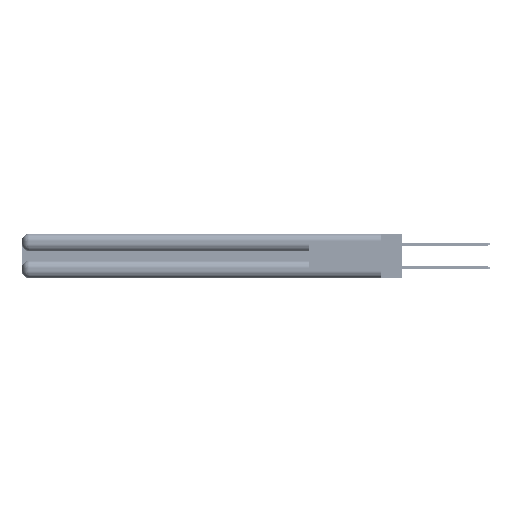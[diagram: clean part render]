
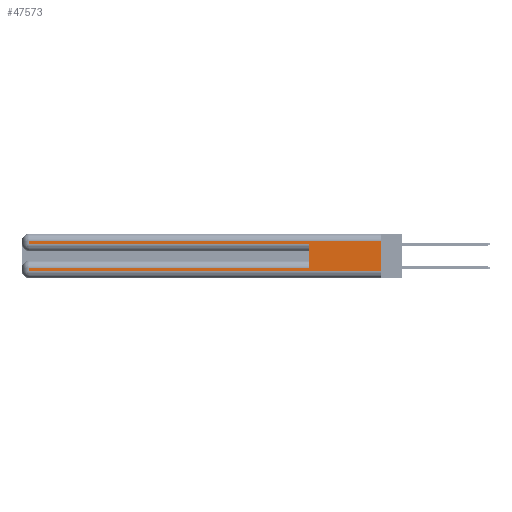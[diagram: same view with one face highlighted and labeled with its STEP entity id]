
A CAD part, left-side view. The second image highlights one B-rep face of the part: STEP entity #47573.
In plain terms, the highlighted planar face has unit normal (-1, 0, 0).
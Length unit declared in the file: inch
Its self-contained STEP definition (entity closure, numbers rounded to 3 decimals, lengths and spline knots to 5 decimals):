
#37 = VECTOR ( 'NONE', #35534, 39.37008 ) ;
#205 = VERTEX_POINT ( 'NONE', #32773 ) ;
#1882 = CARTESIAN_POINT ( 'NONE',  ( 0., 0.6, 0.085 ) ) ;
#2250 = CARTESIAN_POINT ( 'NONE',  ( 0., 2.94, 0.085 ) ) ;
#2563 = EDGE_CURVE ( 'NONE', #205, #37774, #5946, .T. ) ;
#3635 = CARTESIAN_POINT ( 'NONE',  ( 0., 0., 0.285 ) ) ;
#4123 = ORIENTED_EDGE ( 'NONE', *, *, #25211, .F. ) ;
#5076 = VECTOR ( 'NONE', #13682, 39.37008 ) ;
#5824 = EDGE_CURVE ( 'NONE', #36626, #10747, #19608, .T. ) ;
#5946 = LINE ( 'NONE', #14406, #26846 ) ;
#6114 = VERTEX_POINT ( 'NONE', #18124 ) ;
#6304 = CARTESIAN_POINT ( 'NONE',  ( 0., 2.94, 0.37 ) ) ;
#6637 = VECTOR ( 'NONE', #47130, 39.37008 ) ;
#7962 = LINE ( 'NONE', #22402, #6637 ) ;
#8112 = ORIENTED_EDGE ( 'NONE', *, *, #26321, .T. ) ;
#8675 = CARTESIAN_POINT ( 'NONE',  ( 0., 2.94, 0.37 ) ) ;
#10031 = ORIENTED_EDGE ( 'NONE', *, *, #43802, .T. ) ;
#10523 = DIRECTION ( 'NONE',  ( 0., -1., 0. ) ) ;
#10747 = VERTEX_POINT ( 'NONE', #31494 ) ;
#11417 = DIRECTION ( 'NONE',  ( 0., 1., 0. ) ) ;
#12147 = DIRECTION ( 'NONE',  ( 0., -1., 0. ) ) ;
#12159 = LINE ( 'NONE', #44704, #24508 ) ;
#13682 = DIRECTION ( 'NONE',  ( 0., 0., -1. ) ) ;
#13948 = VECTOR ( 'NONE', #46022, 39.37008 ) ;
#14031 = ORIENTED_EDGE ( 'NONE', *, *, #5824, .T. ) ;
#14406 = CARTESIAN_POINT ( 'NONE',  ( 0., 0., 0.06 ) ) ;
#17863 = CARTESIAN_POINT ( 'NONE',  ( 0., 0., 0.37 ) ) ;
#18124 = CARTESIAN_POINT ( 'NONE',  ( 0., 2.94, 0.31 ) ) ;
#19393 = VERTEX_POINT ( 'NONE', #2250 ) ;
#19608 = LINE ( 'NONE', #3635, #30580 ) ;
#19993 = DIRECTION ( 'NONE',  ( 0., 0., 1. ) ) ;
#21186 = ORIENTED_EDGE ( 'NONE', *, *, #26703, .T. ) ;
#22244 = PLANE ( 'NONE',  #25597 ) ;
#22402 = CARTESIAN_POINT ( 'NONE',  ( 0., 0., 0.31 ) ) ;
#22417 = DIRECTION ( 'NONE',  ( 1., 0., 0. ) ) ;
#22661 = CARTESIAN_POINT ( 'NONE',  ( 0., 0., 0.31 ) ) ;
#24508 = VECTOR ( 'NONE', #19993, 39.37008 ) ;
#25211 = EDGE_CURVE ( 'NONE', #25696, #10747, #12159, .T. ) ;
#25597 = AXIS2_PLACEMENT_3D ( 'NONE', #47141, #22417, #51303 ) ;
#25696 = VERTEX_POINT ( 'NONE', #1882 ) ;
#26321 = EDGE_CURVE ( 'NONE', #19393, #205, #33384, .T. ) ;
#26703 = EDGE_CURVE ( 'NONE', #6114, #36626, #46954, .T. ) ;
#26846 = VECTOR ( 'NONE', #10523, 39.37008 ) ;
#28948 = ORIENTED_EDGE ( 'NONE', *, *, #35830, .T. ) ;
#30580 = VECTOR ( 'NONE', #12147, 39.37008 ) ;
#31494 = CARTESIAN_POINT ( 'NONE',  ( 0., 0.6, 0.285 ) ) ;
#32094 = CARTESIAN_POINT ( 'NONE',  ( 0., 0., 0.085 ) ) ;
#32586 = CARTESIAN_POINT ( 'NONE',  ( 0., 0., 0.06 ) ) ;
#32773 = CARTESIAN_POINT ( 'NONE',  ( 0., 2.94, 0.06 ) ) ;
#33384 = LINE ( 'NONE', #6304, #37 ) ;
#35534 = DIRECTION ( 'NONE',  ( 0., 0., -1. ) ) ;
#35830 = EDGE_CURVE ( 'NONE', #25696, #19393, #52358, .T. ) ;
#36626 = VERTEX_POINT ( 'NONE', #53874 ) ;
#37774 = VERTEX_POINT ( 'NONE', #32586 ) ;
#38136 = VERTEX_POINT ( 'NONE', #22661 ) ;
#38221 = LINE ( 'NONE', #17863, #5076 ) ;
#41763 = ORIENTED_EDGE ( 'NONE', *, *, #45667, .F. ) ;
#43802 = EDGE_CURVE ( 'NONE', #38136, #6114, #7962, .T. ) ;
#43922 = VECTOR ( 'NONE', #11417, 39.37008 ) ;
#44704 = CARTESIAN_POINT ( 'NONE',  ( 0., 0.6, 0.145 ) ) ;
#45667 = EDGE_CURVE ( 'NONE', #38136, #37774, #38221, .T. ) ;
#46022 = DIRECTION ( 'NONE',  ( 0., 0., -1. ) ) ;
#46954 = LINE ( 'NONE', #8675, #13948 ) ;
#47130 = DIRECTION ( 'NONE',  ( 0., 1., 0. ) ) ;
#47141 = CARTESIAN_POINT ( 'NONE',  ( 0., 0., 0.37 ) ) ;
#47573 = ADVANCED_FACE ( 'NONE', ( #47772 ), #22244, .F. ) ;
#47723 = EDGE_LOOP ( 'NONE', ( #41763, #10031, #21186, #14031, #4123, #28948, #8112, #52201 ) ) ;
#47772 = FACE_OUTER_BOUND ( 'NONE', #47723, .T. ) ;
#51303 = DIRECTION ( 'NONE',  ( 0., 0., -1. ) ) ;
#52201 = ORIENTED_EDGE ( 'NONE', *, *, #2563, .T. ) ;
#52358 = LINE ( 'NONE', #32094, #43922 ) ;
#53874 = CARTESIAN_POINT ( 'NONE',  ( 0., 2.94, 0.285 ) ) ;
